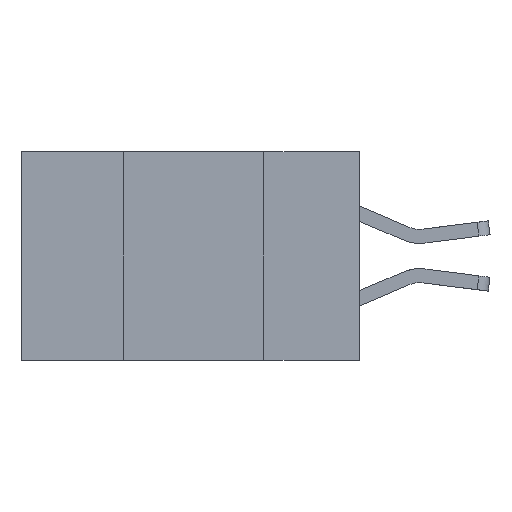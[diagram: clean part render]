
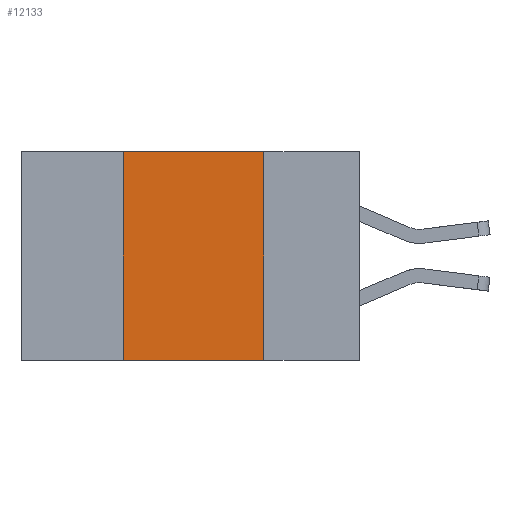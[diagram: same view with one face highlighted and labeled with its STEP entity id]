
A CAD part, left-side view. The second image highlights one B-rep face of the part: STEP entity #12133.
In plain terms, the highlighted planar face has unit normal (-1, 0, 0).
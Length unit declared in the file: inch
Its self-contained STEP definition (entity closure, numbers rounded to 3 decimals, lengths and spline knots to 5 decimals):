
#311 = VECTOR ( 'NONE', #11158, 39.37008 ) ;
#383 = VECTOR ( 'NONE', #5414, 39.37008 ) ;
#743 = LINE ( 'NONE', #12634, #383 ) ;
#805 = LINE ( 'NONE', #6328, #11556 ) ;
#1068 = VERTEX_POINT ( 'NONE', #9017 ) ;
#2242 = CARTESIAN_POINT ( 'NONE',  ( 0., 0.17, -0.37 ) ) ;
#3062 = VECTOR ( 'NONE', #10849, 39.37008 ) ;
#3800 = ORIENTED_EDGE ( 'NONE', *, *, #13275, .F. ) ;
#4432 = CARTESIAN_POINT ( 'NONE',  ( 0., 0.17, 0. ) ) ;
#4530 = PLANE ( 'NONE',  #13343 ) ;
#5414 = DIRECTION ( 'NONE',  ( 0., -1., 0. ) ) ;
#5550 = DIRECTION ( 'NONE',  ( 1., 0., 0. ) ) ;
#6281 = VERTEX_POINT ( 'NONE', #2242 ) ;
#6328 = CARTESIAN_POINT ( 'NONE',  ( 0., 0.17, 0. ) ) ;
#7781 = EDGE_CURVE ( 'NONE', #1068, #6281, #11430, .T. ) ;
#8421 = DIRECTION ( 'NONE',  ( 0., 0., -1. ) ) ;
#9017 = CARTESIAN_POINT ( 'NONE',  ( 0., 0.42, -0.37 ) ) ;
#9299 = EDGE_CURVE ( 'NONE', #12386, #12086, #743, .T. ) ;
#9383 = ORIENTED_EDGE ( 'NONE', *, *, #9299, .F. ) ;
#9824 = CARTESIAN_POINT ( 'NONE',  ( 0., 0.6, -0.37 ) ) ;
#10350 = ORIENTED_EDGE ( 'NONE', *, *, #7781, .T. ) ;
#10849 = DIRECTION ( 'NONE',  ( 0., -1., 0. ) ) ;
#11158 = DIRECTION ( 'NONE',  ( 0., 0., 1. ) ) ;
#11247 = EDGE_CURVE ( 'NONE', #1068, #12386, #11755, .T. ) ;
#11430 = LINE ( 'NONE', #9824, #3062 ) ;
#11556 = VECTOR ( 'NONE', #8421, 39.37008 ) ;
#11746 = CARTESIAN_POINT ( 'NONE',  ( 0., 0.6, 0. ) ) ;
#11755 = LINE ( 'NONE', #13178, #311 ) ;
#12086 = VERTEX_POINT ( 'NONE', #4432 ) ;
#12101 = CARTESIAN_POINT ( 'NONE',  ( 0., 0.42, 0. ) ) ;
#12133 = ADVANCED_FACE ( 'NONE', ( #13453 ), #4530, .F. ) ;
#12386 = VERTEX_POINT ( 'NONE', #12101 ) ;
#12400 = ORIENTED_EDGE ( 'NONE', *, *, #11247, .F. ) ;
#12634 = CARTESIAN_POINT ( 'NONE',  ( 0., 0.6, 0. ) ) ;
#12766 = DIRECTION ( 'NONE',  ( 0., 0., -1. ) ) ;
#13178 = CARTESIAN_POINT ( 'NONE',  ( 0., 0.42, 0. ) ) ;
#13275 = EDGE_CURVE ( 'NONE', #12086, #6281, #805, .T. ) ;
#13343 = AXIS2_PLACEMENT_3D ( 'NONE', #11746, #5550, #12766 ) ;
#13453 = FACE_OUTER_BOUND ( 'NONE', #13807, .T. ) ;
#13807 = EDGE_LOOP ( 'NONE', ( #3800, #9383, #12400, #10350 ) ) ;
